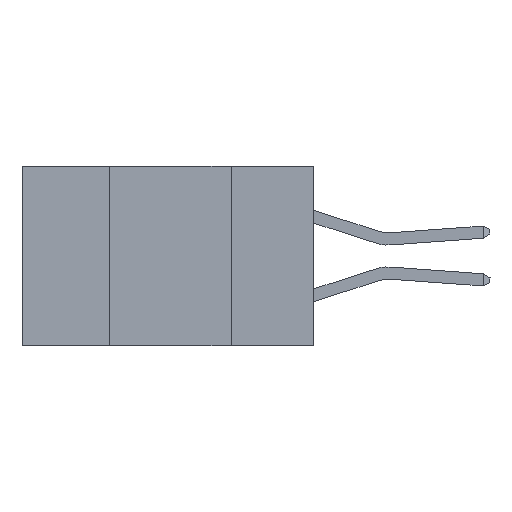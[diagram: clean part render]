
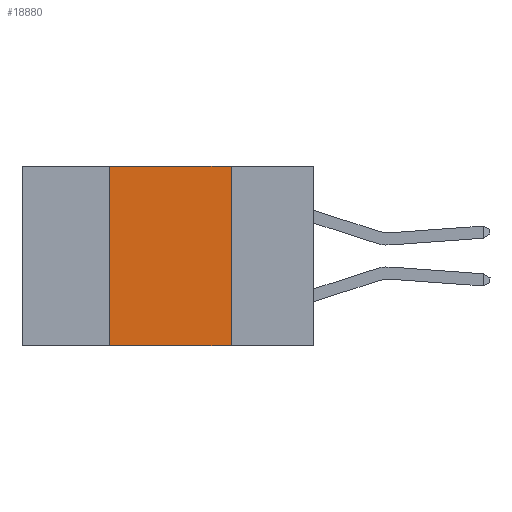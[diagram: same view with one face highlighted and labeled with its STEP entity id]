
A CAD part, left-side view. The second image highlights one B-rep face of the part: STEP entity #18880.
In plain terms, the highlighted planar face has unit normal (-1, 0, 0).
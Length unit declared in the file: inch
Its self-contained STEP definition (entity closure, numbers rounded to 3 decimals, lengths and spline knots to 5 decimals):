
#79 = CARTESIAN_POINT ( 'NONE',  ( 0., 0.42, 0. ) ) ;
#643 = EDGE_CURVE ( 'NONE', #6844, #4850, #18250, .T. ) ;
#1763 = VECTOR ( 'NONE', #19302, 39.37008 ) ;
#1899 = DIRECTION ( 'NONE',  ( 0., 0., -1. ) ) ;
#2029 = DIRECTION ( 'NONE',  ( 0., -1., 0. ) ) ;
#2698 = VECTOR ( 'NONE', #9114, 39.37008 ) ;
#3028 = LINE ( 'NONE', #19433, #10743 ) ;
#3240 = LINE ( 'NONE', #7352, #2698 ) ;
#4775 = DIRECTION ( 'NONE',  ( 0., -1., 0. ) ) ;
#4850 = VERTEX_POINT ( 'NONE', #22380 ) ;
#5620 = CARTESIAN_POINT ( 'NONE',  ( 0., 0.17, 0. ) ) ;
#6536 = EDGE_LOOP ( 'NONE', ( #8952, #11475, #13950, #9789 ) ) ;
#6844 = VERTEX_POINT ( 'NONE', #12750 ) ;
#7140 = CARTESIAN_POINT ( 'NONE',  ( 0., 0.42, 0. ) ) ;
#7352 = CARTESIAN_POINT ( 'NONE',  ( 0., 0.17, 0. ) ) ;
#8912 = PLANE ( 'NONE',  #15063 ) ;
#8952 = ORIENTED_EDGE ( 'NONE', *, *, #15754, .F. ) ;
#8983 = VECTOR ( 'NONE', #4775, 39.37008 ) ;
#9114 = DIRECTION ( 'NONE',  ( 0., 0., -1. ) ) ;
#9789 = ORIENTED_EDGE ( 'NONE', *, *, #643, .T. ) ;
#10675 = CARTESIAN_POINT ( 'NONE',  ( 0., 0.6, 0. ) ) ;
#10743 = VECTOR ( 'NONE', #2029, 39.37008 ) ;
#11400 = FACE_OUTER_BOUND ( 'NONE', #6536, .T. ) ;
#11475 = ORIENTED_EDGE ( 'NONE', *, *, #13887, .F. ) ;
#11574 = CARTESIAN_POINT ( 'NONE',  ( 0., 0.6, -0.37 ) ) ;
#12505 = DIRECTION ( 'NONE',  ( 1., 0., 0. ) ) ;
#12750 = CARTESIAN_POINT ( 'NONE',  ( 0., 0.42, -0.37 ) ) ;
#13887 = EDGE_CURVE ( 'NONE', #17757, #13931, #3028, .T. ) ;
#13931 = VERTEX_POINT ( 'NONE', #5620 ) ;
#13950 = ORIENTED_EDGE ( 'NONE', *, *, #18345, .F. ) ;
#15063 = AXIS2_PLACEMENT_3D ( 'NONE', #10675, #12505, #1899 ) ;
#15754 = EDGE_CURVE ( 'NONE', #13931, #4850, #3240, .T. ) ;
#15819 = LINE ( 'NONE', #7140, #1763 ) ;
#17757 = VERTEX_POINT ( 'NONE', #79 ) ;
#18250 = LINE ( 'NONE', #11574, #8983 ) ;
#18345 = EDGE_CURVE ( 'NONE', #6844, #17757, #15819, .T. ) ;
#18880 = ADVANCED_FACE ( 'NONE', ( #11400 ), #8912, .F. ) ;
#19302 = DIRECTION ( 'NONE',  ( 0., 0., 1. ) ) ;
#19433 = CARTESIAN_POINT ( 'NONE',  ( 0., 0.6, 0. ) ) ;
#22380 = CARTESIAN_POINT ( 'NONE',  ( 0., 0.17, -0.37 ) ) ;
